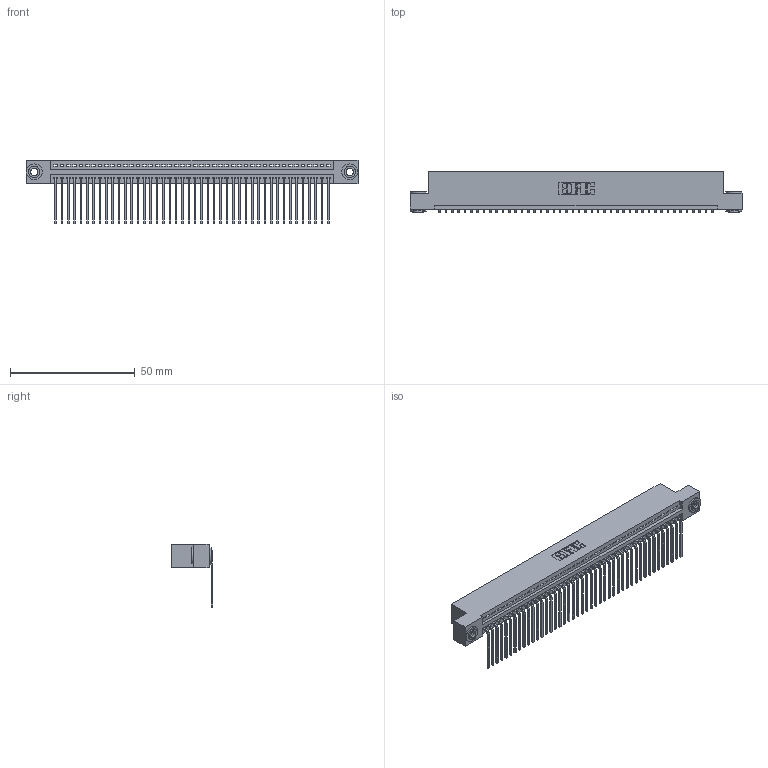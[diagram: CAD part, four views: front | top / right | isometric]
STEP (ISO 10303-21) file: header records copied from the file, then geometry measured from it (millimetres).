
FILE_DESCRIPTION (( 'STEP AP203' ), '1' );
FILE_NAME ('395-044-559-103.STEP', '2019-10-22T17:12:05', ( '' ), ( '' ), 'SwSTEP 2.0', 'SolidWorks 2016', '' );
FILE_SCHEMA (( 'CONFIG_CONTROL_DESIGN' ));
Length unit declared in the file: inch
Products named in the file (4): 395-044-559-103; 345-292-001_558 559 Tail - 1; 345-250-002_345-250-002-102; 345 Part_Flush Mounting Lugs - 0.156 Dia-TH
Assembly tree (47 placements, depth 2):
  395-044-559-103
    345 Part_Flush Mounting Lugs - 0.156 Dia-TH
    345-292-001_558 559 Tail - 1  x44
    345-250-002_345-250-002-102  x2
Bounding box: 132.97 x 16.75 x 25.53 mm (x, y, z)
Volume: 12811.9 mm3; surface area: 18129 mm2
Topology: 47 solids, 47 shells, 2804 faces, 8425 edges, 5554 vertices
Faces by surface type: plane 1938, cylinder 858, cone 8
Entity records: 33580 total; most frequent: CARTESIAN_POINT 5795, ORIENTED_EDGE 5766, DIRECTION 5089, EDGE_CURVE 2883, VECTOR 2551, LINE 2551, VERTEX_POINT 1918, AXIS2_PLACEMENT_3D 1269
